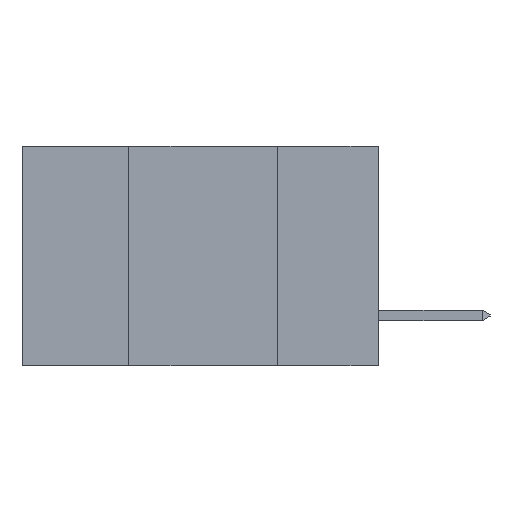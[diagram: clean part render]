
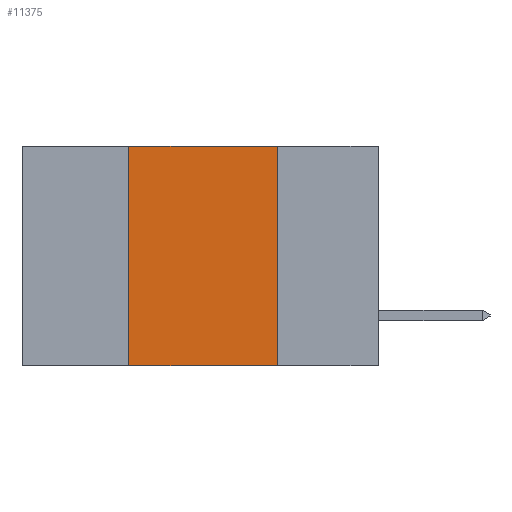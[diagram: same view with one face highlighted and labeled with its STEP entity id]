
A CAD part, left-side view. The second image highlights one B-rep face of the part: STEP entity #11375.
In plain terms, the highlighted planar face has unit normal (-1, 0, 0).
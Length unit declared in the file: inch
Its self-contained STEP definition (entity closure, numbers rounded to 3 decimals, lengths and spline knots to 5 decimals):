
#114 = VECTOR ( 'NONE', #10283, 39.37008 ) ;
#306 = CARTESIAN_POINT ( 'NONE',  ( 0., 0.17, 0. ) ) ;
#1838 = ORIENTED_EDGE ( 'NONE', *, *, #10623, .F. ) ;
#1982 = EDGE_CURVE ( 'NONE', #10731, #9874, #12439, .T. ) ;
#1992 = ORIENTED_EDGE ( 'NONE', *, *, #1982, .F. ) ;
#2400 = PLANE ( 'NONE',  #4974 ) ;
#2571 = ORIENTED_EDGE ( 'NONE', *, *, #5518, .F. ) ;
#2585 = ORIENTED_EDGE ( 'NONE', *, *, #10453, .T. ) ;
#3076 = VERTEX_POINT ( 'NONE', #10748 ) ;
#4595 = DIRECTION ( 'NONE',  ( 1., 0., 0. ) ) ;
#4974 = AXIS2_PLACEMENT_3D ( 'NONE', #8474, #4595, #11354 ) ;
#5518 = EDGE_CURVE ( 'NONE', #3076, #8496, #11001, .T. ) ;
#5590 = DIRECTION ( 'NONE',  ( 0., -1., 0. ) ) ;
#5724 = VECTOR ( 'NONE', #12028, 39.37008 ) ;
#5752 = CARTESIAN_POINT ( 'NONE',  ( 0., 0.17, 0. ) ) ;
#6320 = CARTESIAN_POINT ( 'NONE',  ( 0., 0.6, -0.37 ) ) ;
#6517 = CARTESIAN_POINT ( 'NONE',  ( 0., 0.42, 0. ) ) ;
#6561 = CARTESIAN_POINT ( 'NONE',  ( 0., 0.17, -0.37 ) ) ;
#6698 = DIRECTION ( 'NONE',  ( 0., 0., -1. ) ) ;
#7689 = VECTOR ( 'NONE', #6698, 39.37008 ) ;
#8474 = CARTESIAN_POINT ( 'NONE',  ( 0., 0.6, 0. ) ) ;
#8496 = VERTEX_POINT ( 'NONE', #6517 ) ;
#9874 = VERTEX_POINT ( 'NONE', #6561 ) ;
#10158 = EDGE_LOOP ( 'NONE', ( #1992, #1838, #2571, #2585 ) ) ;
#10283 = DIRECTION ( 'NONE',  ( 0., 0., 1. ) ) ;
#10453 = EDGE_CURVE ( 'NONE', #3076, #9874, #10830, .T. ) ;
#10623 = EDGE_CURVE ( 'NONE', #8496, #10731, #11851, .T. ) ;
#10731 = VERTEX_POINT ( 'NONE', #306 ) ;
#10748 = CARTESIAN_POINT ( 'NONE',  ( 0., 0.42, -0.37 ) ) ;
#10830 = LINE ( 'NONE', #6320, #5724 ) ;
#11001 = LINE ( 'NONE', #12164, #114 ) ;
#11329 = CARTESIAN_POINT ( 'NONE',  ( 0., 0.6, 0. ) ) ;
#11354 = DIRECTION ( 'NONE',  ( 0., 0., -1. ) ) ;
#11375 = ADVANCED_FACE ( 'NONE', ( #11689 ), #2400, .F. ) ;
#11557 = VECTOR ( 'NONE', #5590, 39.37008 ) ;
#11689 = FACE_OUTER_BOUND ( 'NONE', #10158, .T. ) ;
#11851 = LINE ( 'NONE', #11329, #11557 ) ;
#12028 = DIRECTION ( 'NONE',  ( 0., -1., 0. ) ) ;
#12164 = CARTESIAN_POINT ( 'NONE',  ( 0., 0.42, 0. ) ) ;
#12439 = LINE ( 'NONE', #5752, #7689 ) ;
